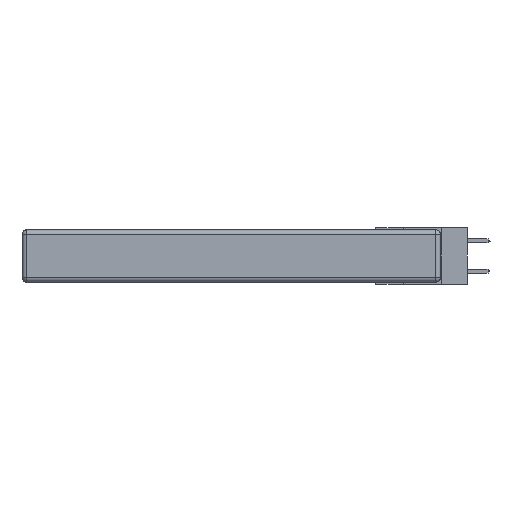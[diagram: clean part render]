
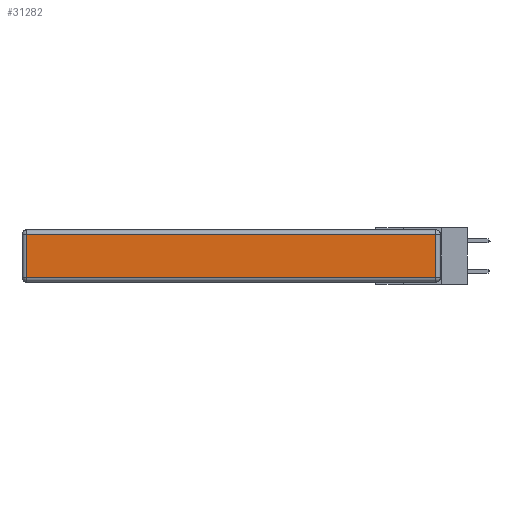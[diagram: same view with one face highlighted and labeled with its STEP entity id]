
A CAD part, left-side view. The second image highlights one B-rep face of the part: STEP entity #31282.
In plain terms, the highlighted planar face has unit normal (-1, 0, 0).
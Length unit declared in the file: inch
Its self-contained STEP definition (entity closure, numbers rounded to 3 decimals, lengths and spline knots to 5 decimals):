
#102 = CARTESIAN_POINT ( 'NONE',  ( 0., 2.72, -0.343 ) ) ;
#1980 = ORIENTED_EDGE ( 'NONE', *, *, #6157, .T. ) ;
#2202 = DIRECTION ( 'NONE',  ( 0., 0., 1. ) ) ;
#2672 = PLANE ( 'NONE',  #12698 ) ;
#2687 = CARTESIAN_POINT ( 'NONE',  ( 0., 2.72, -0.313 ) ) ;
#4440 = ORIENTED_EDGE ( 'NONE', *, *, #9466, .T. ) ;
#5383 = CARTESIAN_POINT ( 'NONE',  ( 0., 0., -0.343 ) ) ;
#5483 = DIRECTION ( 'NONE',  ( 0., 0., -1. ) ) ;
#6157 = EDGE_CURVE ( 'NONE', #22374, #27605, #24712, .T. ) ;
#6222 = LINE ( 'NONE', #20136, #32422 ) ;
#6358 = FACE_OUTER_BOUND ( 'NONE', #18734, .T. ) ;
#7224 = LINE ( 'NONE', #28706, #27528 ) ;
#7473 = LINE ( 'NONE', #10085, #17827 ) ;
#8897 = CARTESIAN_POINT ( 'NONE',  ( 0., 0.03, -0.03 ) ) ;
#9466 = EDGE_CURVE ( 'NONE', #18038, #25953, #6222, .T. ) ;
#10085 = CARTESIAN_POINT ( 'NONE',  ( 0., 2.75, -0.03 ) ) ;
#10302 = DIRECTION ( 'NONE',  ( 0., 0., 1. ) ) ;
#11144 = CARTESIAN_POINT ( 'NONE',  ( 0., 2.72, -0.03 ) ) ;
#12698 = AXIS2_PLACEMENT_3D ( 'NONE', #5383, #25511, #10302 ) ;
#13284 = EDGE_CURVE ( 'NONE', #25953, #22374, #7473, .T. ) ;
#14408 = VECTOR ( 'NONE', #5483, 39.37008 ) ;
#15060 = ORIENTED_EDGE ( 'NONE', *, *, #13284, .T. ) ;
#15192 = CARTESIAN_POINT ( 'NONE',  ( 0., 0.03, -0.313 ) ) ;
#15325 = DIRECTION ( 'NONE',  ( 0., 1., 0. ) ) ;
#15903 = ORIENTED_EDGE ( 'NONE', *, *, #16363, .T. ) ;
#16363 = EDGE_CURVE ( 'NONE', #27605, #18038, #7224, .T. ) ;
#17827 = VECTOR ( 'NONE', #15325, 39.37008 ) ;
#18038 = VERTEX_POINT ( 'NONE', #15192 ) ;
#18206 = DIRECTION ( 'NONE',  ( 0., -1., 0. ) ) ;
#18734 = EDGE_LOOP ( 'NONE', ( #15903, #4440, #15060, #1980 ) ) ;
#20136 = CARTESIAN_POINT ( 'NONE',  ( 0., 0.03, -0.343 ) ) ;
#22374 = VERTEX_POINT ( 'NONE', #11144 ) ;
#24712 = LINE ( 'NONE', #102, #14408 ) ;
#25511 = DIRECTION ( 'NONE',  ( -1., 0., 0. ) ) ;
#25953 = VERTEX_POINT ( 'NONE', #8897 ) ;
#27528 = VECTOR ( 'NONE', #18206, 39.37008 ) ;
#27605 = VERTEX_POINT ( 'NONE', #2687 ) ;
#28706 = CARTESIAN_POINT ( 'NONE',  ( 0., 0., -0.313 ) ) ;
#31282 = ADVANCED_FACE ( 'NONE', ( #6358 ), #2672, .T. ) ;
#32422 = VECTOR ( 'NONE', #2202, 39.37008 ) ;
